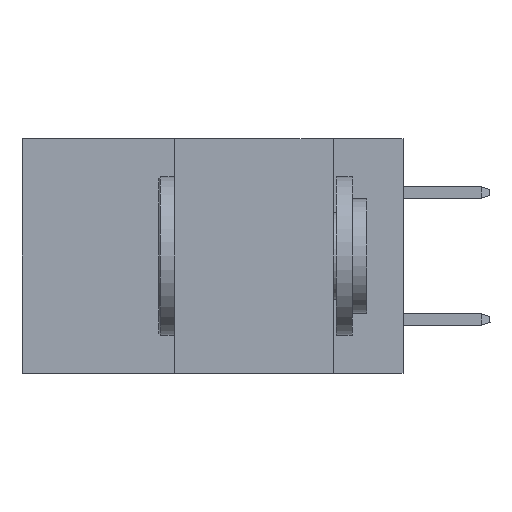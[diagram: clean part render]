
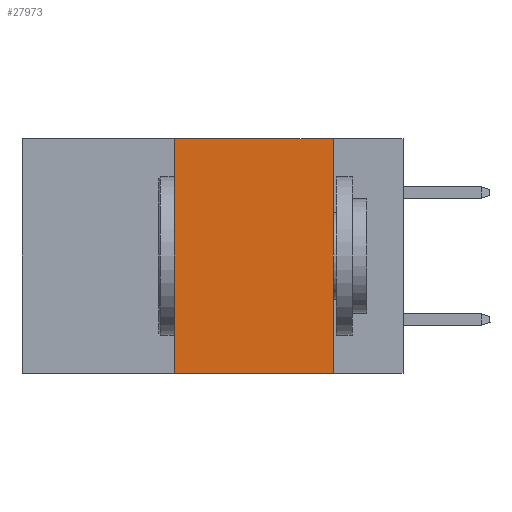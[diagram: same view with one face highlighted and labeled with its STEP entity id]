
A CAD part, left-side view. The second image highlights one B-rep face of the part: STEP entity #27973.
In plain terms, the highlighted planar face has unit normal (-1, 0, 0).
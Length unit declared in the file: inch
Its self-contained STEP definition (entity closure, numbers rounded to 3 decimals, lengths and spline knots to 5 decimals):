
#1568 = DIRECTION ( 'NONE',  ( 0., 0., -1. ) ) ;
#1782 = ORIENTED_EDGE ( 'NONE', *, *, #21648, .F. ) ;
#1967 = ORIENTED_EDGE ( 'NONE', *, *, #17297, .F. ) ;
#1972 = CARTESIAN_POINT ( 'NONE',  ( 0., 0.36, 0. ) ) ;
#5387 = EDGE_CURVE ( 'NONE', #16962, #16854, #12451, .T. ) ;
#5443 = DIRECTION ( 'NONE',  ( 0., -1., 0. ) ) ;
#7171 = CARTESIAN_POINT ( 'NONE',  ( 0., 0.36, 0. ) ) ;
#7418 = LINE ( 'NONE', #22141, #27078 ) ;
#9139 = VERTEX_POINT ( 'NONE', #23748 ) ;
#9730 = VECTOR ( 'NONE', #5443, 39.37008 ) ;
#9782 = DIRECTION ( 'NONE',  ( 0., -1., 0. ) ) ;
#10200 = CARTESIAN_POINT ( 'NONE',  ( 0., 0.6, 0. ) ) ;
#10604 = DIRECTION ( 'NONE',  ( 0., 0., 1. ) ) ;
#11237 = ORIENTED_EDGE ( 'NONE', *, *, #5387, .F. ) ;
#11479 = CARTESIAN_POINT ( 'NONE',  ( 0., 0.6, -0.37 ) ) ;
#11774 = DIRECTION ( 'NONE',  ( 0., 0., -1. ) ) ;
#12040 = LINE ( 'NONE', #11479, #22023 ) ;
#12451 = LINE ( 'NONE', #1972, #22166 ) ;
#14407 = AXIS2_PLACEMENT_3D ( 'NONE', #10200, #20838, #1568 ) ;
#14731 = EDGE_CURVE ( 'NONE', #16962, #9139, #12040, .T. ) ;
#16481 = CARTESIAN_POINT ( 'NONE',  ( 0., 0.36, -0.37 ) ) ;
#16854 = VERTEX_POINT ( 'NONE', #7171 ) ;
#16962 = VERTEX_POINT ( 'NONE', #16481 ) ;
#17087 = EDGE_LOOP ( 'NONE', ( #1967, #1782, #11237, #24037 ) ) ;
#17297 = EDGE_CURVE ( 'NONE', #24042, #9139, #7418, .T. ) ;
#19346 = CARTESIAN_POINT ( 'NONE',  ( 0., 0.11, 0. ) ) ;
#20838 = DIRECTION ( 'NONE',  ( 1., 0., 0. ) ) ;
#21648 = EDGE_CURVE ( 'NONE', #16854, #24042, #27380, .T. ) ;
#22023 = VECTOR ( 'NONE', #9782, 39.37008 ) ;
#22141 = CARTESIAN_POINT ( 'NONE',  ( 0., 0.11, 0. ) ) ;
#22166 = VECTOR ( 'NONE', #10604, 39.37008 ) ;
#23142 = CARTESIAN_POINT ( 'NONE',  ( 0., 0.6, 0. ) ) ;
#23244 = FACE_OUTER_BOUND ( 'NONE', #17087, .T. ) ;
#23748 = CARTESIAN_POINT ( 'NONE',  ( 0., 0.11, -0.37 ) ) ;
#24037 = ORIENTED_EDGE ( 'NONE', *, *, #14731, .T. ) ;
#24042 = VERTEX_POINT ( 'NONE', #19346 ) ;
#27078 = VECTOR ( 'NONE', #11774, 39.37008 ) ;
#27196 = PLANE ( 'NONE',  #14407 ) ;
#27380 = LINE ( 'NONE', #23142, #9730 ) ;
#27973 = ADVANCED_FACE ( 'NONE', ( #23244 ), #27196, .F. ) ;
